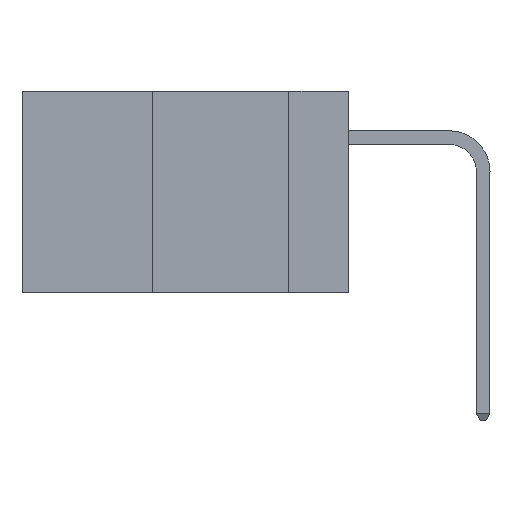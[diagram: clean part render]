
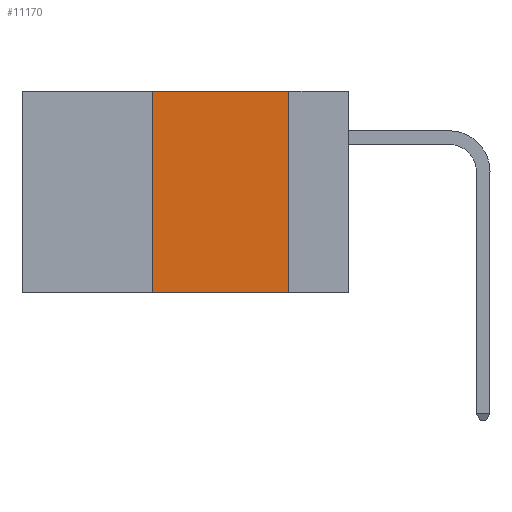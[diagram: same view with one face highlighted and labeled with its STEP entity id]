
A CAD part, left-side view. The second image highlights one B-rep face of the part: STEP entity #11170.
In plain terms, the highlighted planar face has unit normal (-1, 0, 0).
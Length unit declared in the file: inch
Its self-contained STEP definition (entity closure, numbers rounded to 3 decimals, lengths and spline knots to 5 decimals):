
#494 = DIRECTION ( 'NONE',  ( 0., 0., 1. ) ) ;
#530 = VERTEX_POINT ( 'NONE', #6590 ) ;
#1803 = EDGE_CURVE ( 'NONE', #16848, #530, #26533, .T. ) ;
#2118 = CARTESIAN_POINT ( 'NONE',  ( 0., 0.6, -0.37 ) ) ;
#5163 = DIRECTION ( 'NONE',  ( 0., -1., 0. ) ) ;
#6590 = CARTESIAN_POINT ( 'NONE',  ( 0., 0.11, 0. ) ) ;
#6615 = VECTOR ( 'NONE', #494, 39.37008 ) ;
#6630 = DIRECTION ( 'NONE',  ( 1., 0., 0. ) ) ;
#8096 = CARTESIAN_POINT ( 'NONE',  ( 0., 0.11, -0.37 ) ) ;
#9593 = CARTESIAN_POINT ( 'NONE',  ( 0., 0.6, 0. ) ) ;
#11152 = EDGE_CURVE ( 'NONE', #22901, #16848, #32172, .T. ) ;
#11170 = ADVANCED_FACE ( 'NONE', ( #38386 ), #25095, .F. ) ;
#11918 = EDGE_CURVE ( 'NONE', #22901, #33217, #18575, .T. ) ;
#12785 = AXIS2_PLACEMENT_3D ( 'NONE', #9593, #6630, #28160 ) ;
#14998 = ORIENTED_EDGE ( 'NONE', *, *, #1803, .F. ) ;
#15750 = CARTESIAN_POINT ( 'NONE',  ( 0., 0.6, 0. ) ) ;
#16848 = VERTEX_POINT ( 'NONE', #26681 ) ;
#16885 = LINE ( 'NONE', #25886, #32335 ) ;
#18320 = VECTOR ( 'NONE', #18863, 39.37008 ) ;
#18575 = LINE ( 'NONE', #2118, #34011 ) ;
#18863 = DIRECTION ( 'NONE',  ( 0., -1., 0. ) ) ;
#22901 = VERTEX_POINT ( 'NONE', #24960 ) ;
#24960 = CARTESIAN_POINT ( 'NONE',  ( 0., 0.36, -0.37 ) ) ;
#25095 = PLANE ( 'NONE',  #12785 ) ;
#25886 = CARTESIAN_POINT ( 'NONE',  ( 0., 0.11, 0. ) ) ;
#26533 = LINE ( 'NONE', #15750, #18320 ) ;
#26681 = CARTESIAN_POINT ( 'NONE',  ( 0., 0.36, 0. ) ) ;
#28160 = DIRECTION ( 'NONE',  ( 0., 0., -1. ) ) ;
#28671 = ORIENTED_EDGE ( 'NONE', *, *, #11918, .T. ) ;
#28968 = DIRECTION ( 'NONE',  ( 0., 0., -1. ) ) ;
#32172 = LINE ( 'NONE', #37314, #6615 ) ;
#32335 = VECTOR ( 'NONE', #28968, 39.37008 ) ;
#33217 = VERTEX_POINT ( 'NONE', #8096 ) ;
#33752 = EDGE_LOOP ( 'NONE', ( #38155, #14998, #35474, #28671 ) ) ;
#34011 = VECTOR ( 'NONE', #5163, 39.37008 ) ;
#34928 = EDGE_CURVE ( 'NONE', #530, #33217, #16885, .T. ) ;
#35474 = ORIENTED_EDGE ( 'NONE', *, *, #11152, .F. ) ;
#37314 = CARTESIAN_POINT ( 'NONE',  ( 0., 0.36, 0. ) ) ;
#38155 = ORIENTED_EDGE ( 'NONE', *, *, #34928, .F. ) ;
#38386 = FACE_OUTER_BOUND ( 'NONE', #33752, .T. ) ;
